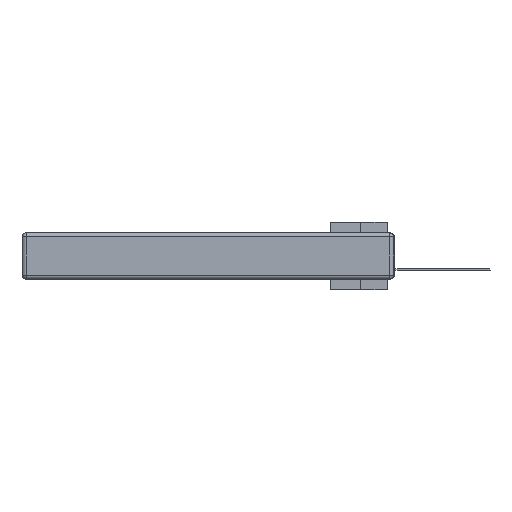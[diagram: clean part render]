
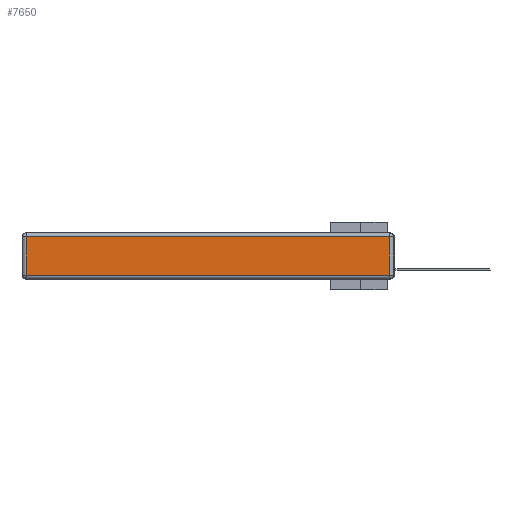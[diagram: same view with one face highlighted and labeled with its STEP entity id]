
A CAD part, left-side view. The second image highlights one B-rep face of the part: STEP entity #7650.
In plain terms, the highlighted planar face has unit normal (-1, 0, 0).
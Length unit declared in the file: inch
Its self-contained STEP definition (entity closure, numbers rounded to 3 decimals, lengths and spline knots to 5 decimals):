
#357 = VECTOR ( 'NONE', #27452, 39.37008 ) ;
#375 = DIRECTION ( 'NONE',  ( 0., 0., 1. ) ) ;
#1795 = VERTEX_POINT ( 'NONE', #2976 ) ;
#1912 = LINE ( 'NONE', #10770, #26340 ) ;
#2862 = EDGE_CURVE ( 'NONE', #1795, #22835, #16378, .T. ) ;
#2976 = CARTESIAN_POINT ( 'NONE',  ( 0., 2.72, -0.03 ) ) ;
#3713 = DIRECTION ( 'NONE',  ( 0., 0., 1. ) ) ;
#3777 = LINE ( 'NONE', #28612, #9005 ) ;
#6437 = CARTESIAN_POINT ( 'NONE',  ( 0., 0.03, -0.313 ) ) ;
#6678 = LINE ( 'NONE', #11127, #357 ) ;
#7382 = VERTEX_POINT ( 'NONE', #6437 ) ;
#7650 = ADVANCED_FACE ( 'NONE', ( #20397 ), #19283, .T. ) ;
#8492 = ORIENTED_EDGE ( 'NONE', *, *, #25740, .T. ) ;
#9005 = VECTOR ( 'NONE', #23659, 39.37008 ) ;
#9040 = VECTOR ( 'NONE', #20717, 39.37008 ) ;
#10770 = CARTESIAN_POINT ( 'NONE',  ( 0., 0.03, -0.343 ) ) ;
#11127 = CARTESIAN_POINT ( 'NONE',  ( 0., 0., -0.313 ) ) ;
#11309 = ORIENTED_EDGE ( 'NONE', *, *, #11610, .T. ) ;
#11525 = ORIENTED_EDGE ( 'NONE', *, *, #2862, .T. ) ;
#11610 = EDGE_CURVE ( 'NONE', #22835, #7382, #6678, .T. ) ;
#14542 = CARTESIAN_POINT ( 'NONE',  ( 0., 0., -0.343 ) ) ;
#15640 = EDGE_CURVE ( 'NONE', #7382, #16303, #1912, .T. ) ;
#16303 = VERTEX_POINT ( 'NONE', #24458 ) ;
#16378 = LINE ( 'NONE', #25295, #9040 ) ;
#19283 = PLANE ( 'NONE',  #20906 ) ;
#19766 = EDGE_LOOP ( 'NONE', ( #11309, #22242, #8492, #11525 ) ) ;
#20397 = FACE_OUTER_BOUND ( 'NONE', #19766, .T. ) ;
#20717 = DIRECTION ( 'NONE',  ( 0., 0., -1. ) ) ;
#20906 = AXIS2_PLACEMENT_3D ( 'NONE', #14542, #28619, #375 ) ;
#22242 = ORIENTED_EDGE ( 'NONE', *, *, #15640, .T. ) ;
#22835 = VERTEX_POINT ( 'NONE', #29213 ) ;
#23659 = DIRECTION ( 'NONE',  ( 0., 1., 0. ) ) ;
#24458 = CARTESIAN_POINT ( 'NONE',  ( 0., 0.03, -0.03 ) ) ;
#25295 = CARTESIAN_POINT ( 'NONE',  ( 0., 2.72, -0.343 ) ) ;
#25740 = EDGE_CURVE ( 'NONE', #16303, #1795, #3777, .T. ) ;
#26340 = VECTOR ( 'NONE', #3713, 39.37008 ) ;
#27452 = DIRECTION ( 'NONE',  ( 0., -1., 0. ) ) ;
#28612 = CARTESIAN_POINT ( 'NONE',  ( 0., 2.75, -0.03 ) ) ;
#28619 = DIRECTION ( 'NONE',  ( -1., 0., 0. ) ) ;
#29213 = CARTESIAN_POINT ( 'NONE',  ( 0., 2.72, -0.313 ) ) ;
